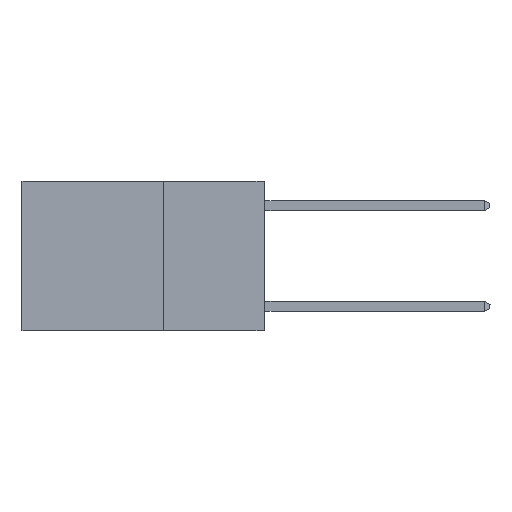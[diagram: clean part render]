
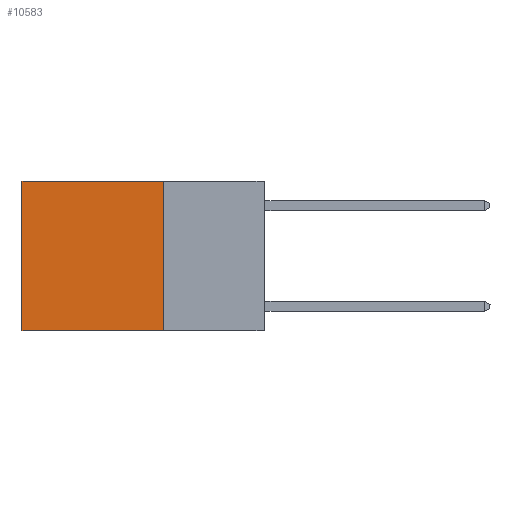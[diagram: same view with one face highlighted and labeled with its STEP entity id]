
A CAD part, left-side view. The second image highlights one B-rep face of the part: STEP entity #10583.
In plain terms, the highlighted planar face has unit normal (-1, 0, 0).
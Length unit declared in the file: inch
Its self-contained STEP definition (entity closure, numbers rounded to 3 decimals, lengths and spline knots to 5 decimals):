
#351 = EDGE_CURVE ( 'NONE', #3816, #6635, #10843, .T. ) ;
#371 = FACE_OUTER_BOUND ( 'NONE', #3596, .T. ) ;
#468 = VECTOR ( 'NONE', #1136, 39.37008 ) ;
#515 = EDGE_CURVE ( 'NONE', #11873, #6635, #3394, .T. ) ;
#1136 = DIRECTION ( 'NONE',  ( 0., 0., -1. ) ) ;
#1815 = CARTESIAN_POINT ( 'NONE',  ( 0.2625, 0.25, 0. ) ) ;
#1864 = PLANE ( 'NONE',  #4742 ) ;
#2006 = DIRECTION ( 'NONE',  ( 0., 0., -1. ) ) ;
#2666 = CARTESIAN_POINT ( 'NONE',  ( 0.2625, 0.25, 0. ) ) ;
#2956 = DIRECTION ( 'NONE',  ( 0., 0., -1. ) ) ;
#3394 = LINE ( 'NONE', #6570, #468 ) ;
#3596 = EDGE_LOOP ( 'NONE', ( #9514, #12382, #4448, #7346 ) ) ;
#3816 = VERTEX_POINT ( 'NONE', #12449 ) ;
#4448 = ORIENTED_EDGE ( 'NONE', *, *, #5558, .F. ) ;
#4742 = AXIS2_PLACEMENT_3D ( 'NONE', #1815, #9448, #2956 ) ;
#4941 = CARTESIAN_POINT ( 'NONE',  ( 0.2625, 0.6, -0.37 ) ) ;
#5134 = EDGE_CURVE ( 'NONE', #11237, #11873, #8901, .T. ) ;
#5558 = EDGE_CURVE ( 'NONE', #11237, #3816, #8884, .T. ) ;
#6000 = VECTOR ( 'NONE', #2006, 39.37008 ) ;
#6570 = CARTESIAN_POINT ( 'NONE',  ( 0.2625, 0.6, 0. ) ) ;
#6635 = VERTEX_POINT ( 'NONE', #4941 ) ;
#7346 = ORIENTED_EDGE ( 'NONE', *, *, #5134, .T. ) ;
#7724 = CARTESIAN_POINT ( 'NONE',  ( 0.2625, 0.6, 0. ) ) ;
#8007 = VECTOR ( 'NONE', #11401, 39.37008 ) ;
#8149 = CARTESIAN_POINT ( 'NONE',  ( 0.2625, 0.25, -0.37 ) ) ;
#8220 = VECTOR ( 'NONE', #9261, 39.37008 ) ;
#8884 = LINE ( 'NONE', #13883, #6000 ) ;
#8901 = LINE ( 'NONE', #2666, #8220 ) ;
#9261 = DIRECTION ( 'NONE',  ( 0., 1., 0. ) ) ;
#9448 = DIRECTION ( 'NONE',  ( 1., 0., 0. ) ) ;
#9514 = ORIENTED_EDGE ( 'NONE', *, *, #515, .T. ) ;
#10583 = ADVANCED_FACE ( 'NONE', ( #371 ), #1864, .F. ) ;
#10843 = LINE ( 'NONE', #8149, #8007 ) ;
#11237 = VERTEX_POINT ( 'NONE', #13835 ) ;
#11401 = DIRECTION ( 'NONE',  ( 0., 1., 0. ) ) ;
#11873 = VERTEX_POINT ( 'NONE', #7724 ) ;
#12382 = ORIENTED_EDGE ( 'NONE', *, *, #351, .F. ) ;
#12449 = CARTESIAN_POINT ( 'NONE',  ( 0.2625, 0.25, -0.37 ) ) ;
#13835 = CARTESIAN_POINT ( 'NONE',  ( 0.2625, 0.25, 0. ) ) ;
#13883 = CARTESIAN_POINT ( 'NONE',  ( 0.2625, 0.25, 0. ) ) ;
